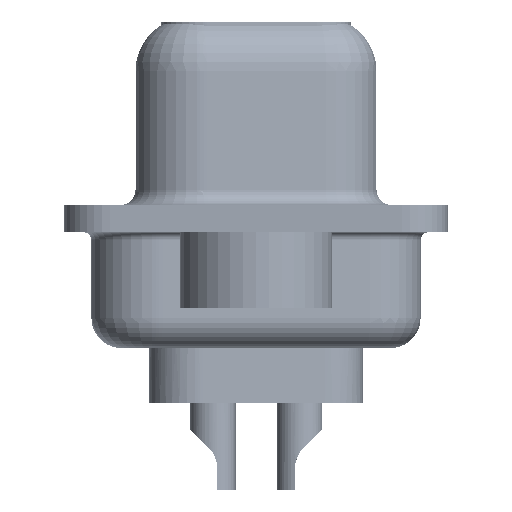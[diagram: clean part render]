
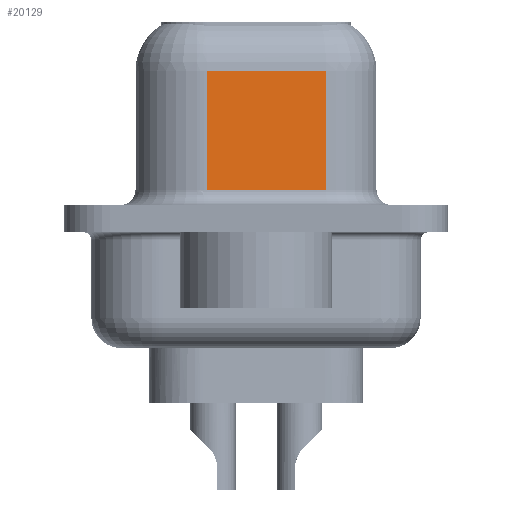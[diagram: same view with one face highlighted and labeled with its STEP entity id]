
A CAD part, left-side view. The second image highlights one B-rep face of the part: STEP entity #20129.
In plain terms, the highlighted planar face has unit normal (-0.985, -0.174, 0).
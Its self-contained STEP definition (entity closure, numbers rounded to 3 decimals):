
#350 = CARTESIAN_POINT ( 'NONE',  ( 5.068, -2.297, 0.95 ) ) ;
#522 = ORIENTED_EDGE ( 'NONE', *, *, #8403, .T. ) ;
#1892 = ORIENTED_EDGE ( 'NONE', *, *, #5924, .T. ) ;
#4371 = LINE ( 'NONE', #27617, #15556 ) ;
#5527 = ORIENTED_EDGE ( 'NONE', *, *, #19533, .T. ) ;
#5924 = EDGE_CURVE ( 'NONE', #15889, #6312, #4371, .T. ) ;
#6028 = EDGE_CURVE ( 'NONE', #19819, #25496, #18752, .T. ) ;
#6230 = DIRECTION ( 'NONE',  ( 0.174, -0.985, 0. ) ) ;
#6312 = VERTEX_POINT ( 'NONE', #25861 ) ;
#6683 = DIRECTION ( 'NONE',  ( 0., 0., -1. ) ) ;
#6991 = AXIS2_PLACEMENT_3D ( 'NONE', #20662, #9942, #21423 ) ;
#7404 = EDGE_LOOP ( 'NONE', ( #28060, #522, #1892, #5527 ) ) ;
#8403 = EDGE_CURVE ( 'NONE', #19819, #15889, #8980, .T. ) ;
#8520 = LINE ( 'NONE', #17858, #23058 ) ;
#8980 = LINE ( 'NONE', #13743, #17854 ) ;
#9280 = DIRECTION ( 'NONE',  ( 0., 0., -1. ) ) ;
#9942 = DIRECTION ( 'NONE',  ( 0.985, 0.174, 0. ) ) ;
#11341 = PLANE ( 'NONE',  #6991 ) ;
#13743 = CARTESIAN_POINT ( 'NONE',  ( 5.068, -2.297, 4.85 ) ) ;
#14581 = CARTESIAN_POINT ( 'NONE',  ( 4.38, 1.603, 4.85 ) ) ;
#15556 = VECTOR ( 'NONE', #6683, 1000. ) ;
#15889 = VERTEX_POINT ( 'NONE', #14581 ) ;
#17854 = VECTOR ( 'NONE', #20315, 1000. ) ;
#17858 = CARTESIAN_POINT ( 'NONE',  ( 5.068, -2.297, 0.95 ) ) ;
#18752 = LINE ( 'NONE', #25779, #27746 ) ;
#19533 = EDGE_CURVE ( 'NONE', #6312, #25496, #8520, .T. ) ;
#19819 = VERTEX_POINT ( 'NONE', #24532 ) ;
#20129 = ADVANCED_FACE ( 'NONE', ( #22964 ), #11341, .F. ) ;
#20315 = DIRECTION ( 'NONE',  ( -0.174, 0.985, 0. ) ) ;
#20662 = CARTESIAN_POINT ( 'NONE',  ( 5.068, -2.297, 6.6 ) ) ;
#21423 = DIRECTION ( 'NONE',  ( -0.174, 0.985, 0. ) ) ;
#22964 = FACE_OUTER_BOUND ( 'NONE', #7404, .T. ) ;
#23058 = VECTOR ( 'NONE', #6230, 1000. ) ;
#24532 = CARTESIAN_POINT ( 'NONE',  ( 5.068, -2.297, 4.85 ) ) ;
#25496 = VERTEX_POINT ( 'NONE', #350 ) ;
#25779 = CARTESIAN_POINT ( 'NONE',  ( 5.068, -2.297, 6.6 ) ) ;
#25861 = CARTESIAN_POINT ( 'NONE',  ( 4.38, 1.603, 0.95 ) ) ;
#27617 = CARTESIAN_POINT ( 'NONE',  ( 4.38, 1.603, 6.6 ) ) ;
#27746 = VECTOR ( 'NONE', #9280, 1000. ) ;
#28060 = ORIENTED_EDGE ( 'NONE', *, *, #6028, .F. ) ;
